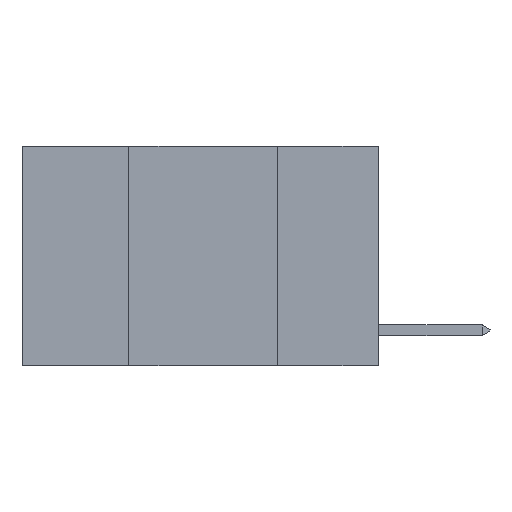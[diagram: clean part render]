
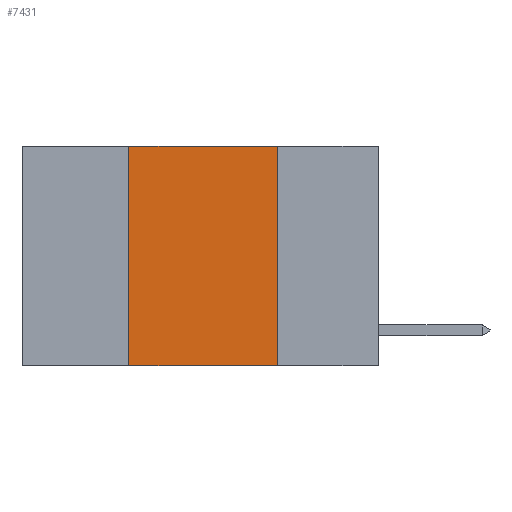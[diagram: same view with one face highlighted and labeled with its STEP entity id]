
A CAD part, left-side view. The second image highlights one B-rep face of the part: STEP entity #7431.
In plain terms, the highlighted planar face has unit normal (-1, 0, 0).
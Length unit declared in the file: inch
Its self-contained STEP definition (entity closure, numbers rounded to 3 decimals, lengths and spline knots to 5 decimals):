
#869 = VECTOR ( 'NONE', #12113, 39.37008 ) ;
#919 = ORIENTED_EDGE ( 'NONE', *, *, #9319, .T. ) ;
#1292 = LINE ( 'NONE', #11011, #869 ) ;
#1912 = PLANE ( 'NONE',  #7233 ) ;
#2203 = EDGE_CURVE ( 'NONE', #9954, #14757, #11798, .T. ) ;
#2359 = CARTESIAN_POINT ( 'NONE',  ( 0., 0.42, 0. ) ) ;
#3094 = CARTESIAN_POINT ( 'NONE',  ( 0., 0.17, 0. ) ) ;
#3099 = DIRECTION ( 'NONE',  ( 0., 0., -1. ) ) ;
#4194 = DIRECTION ( 'NONE',  ( 0., -1., 0. ) ) ;
#5322 = VECTOR ( 'NONE', #7723, 39.37008 ) ;
#5562 = EDGE_LOOP ( 'NONE', ( #8803, #6500, #12832, #919 ) ) ;
#5635 = CARTESIAN_POINT ( 'NONE',  ( 0., 0.17, 0. ) ) ;
#6500 = ORIENTED_EDGE ( 'NONE', *, *, #2203, .F. ) ;
#6520 = VERTEX_POINT ( 'NONE', #12846 ) ;
#7233 = AXIS2_PLACEMENT_3D ( 'NONE', #14315, #9961, #3099 ) ;
#7431 = ADVANCED_FACE ( 'NONE', ( #10592 ), #1912, .F. ) ;
#7723 = DIRECTION ( 'NONE',  ( 0., 0., -1. ) ) ;
#8776 = LINE ( 'NONE', #2359, #14638 ) ;
#8803 = ORIENTED_EDGE ( 'NONE', *, *, #11576, .F. ) ;
#8854 = EDGE_CURVE ( 'NONE', #6520, #9954, #8776, .T. ) ;
#9319 = EDGE_CURVE ( 'NONE', #6520, #10319, #1292, .T. ) ;
#9954 = VERTEX_POINT ( 'NONE', #14504 ) ;
#9961 = DIRECTION ( 'NONE',  ( 1., 0., 0. ) ) ;
#10319 = VERTEX_POINT ( 'NONE', #12822 ) ;
#10399 = DIRECTION ( 'NONE',  ( 0., 0., 1. ) ) ;
#10592 = FACE_OUTER_BOUND ( 'NONE', #5562, .T. ) ;
#11011 = CARTESIAN_POINT ( 'NONE',  ( 0., 0.6, -0.37 ) ) ;
#11115 = VECTOR ( 'NONE', #4194, 39.37008 ) ;
#11576 = EDGE_CURVE ( 'NONE', #14757, #10319, #14224, .T. ) ;
#11798 = LINE ( 'NONE', #12124, #11115 ) ;
#12113 = DIRECTION ( 'NONE',  ( 0., -1., 0. ) ) ;
#12124 = CARTESIAN_POINT ( 'NONE',  ( 0., 0.6, 0. ) ) ;
#12822 = CARTESIAN_POINT ( 'NONE',  ( 0., 0.17, -0.37 ) ) ;
#12832 = ORIENTED_EDGE ( 'NONE', *, *, #8854, .F. ) ;
#12846 = CARTESIAN_POINT ( 'NONE',  ( 0., 0.42, -0.37 ) ) ;
#14224 = LINE ( 'NONE', #3094, #5322 ) ;
#14315 = CARTESIAN_POINT ( 'NONE',  ( 0., 0.6, 0. ) ) ;
#14504 = CARTESIAN_POINT ( 'NONE',  ( 0., 0.42, 0. ) ) ;
#14638 = VECTOR ( 'NONE', #10399, 39.37008 ) ;
#14757 = VERTEX_POINT ( 'NONE', #5635 ) ;
